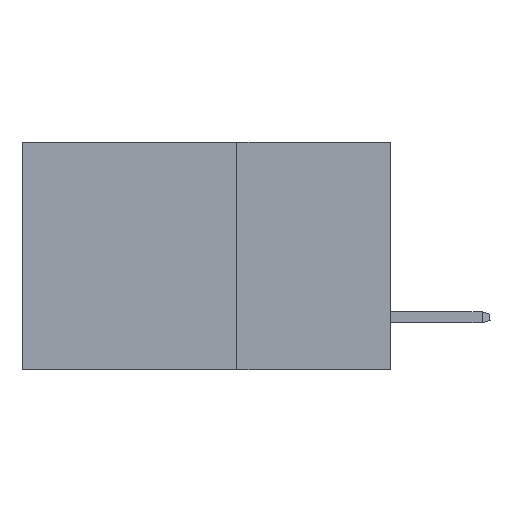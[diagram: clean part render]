
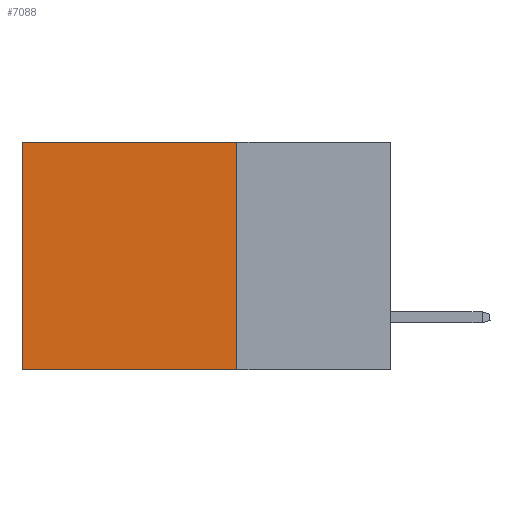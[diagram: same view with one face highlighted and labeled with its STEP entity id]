
A CAD part, left-side view. The second image highlights one B-rep face of the part: STEP entity #7088.
In plain terms, the highlighted planar face has unit normal (-1, 0, 0).
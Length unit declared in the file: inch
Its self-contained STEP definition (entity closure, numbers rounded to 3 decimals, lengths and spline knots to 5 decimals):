
#623 = CARTESIAN_POINT ( 'NONE',  ( 0.2875, 0.25, 0. ) ) ;
#876 = VECTOR ( 'NONE', #15731, 39.37008 ) ;
#918 = CARTESIAN_POINT ( 'NONE',  ( 0.2875, 0.25, 0. ) ) ;
#2680 = CARTESIAN_POINT ( 'NONE',  ( 0.2875, 0.6, 0. ) ) ;
#2746 = CARTESIAN_POINT ( 'NONE',  ( 0.2875, 0.6, -0.37 ) ) ;
#3376 = LINE ( 'NONE', #7480, #18117 ) ;
#4054 = VERTEX_POINT ( 'NONE', #22107 ) ;
#5449 = EDGE_CURVE ( 'NONE', #4054, #9744, #11555, .T. ) ;
#5782 = PLANE ( 'NONE',  #20547 ) ;
#7088 = ADVANCED_FACE ( 'NONE', ( #18167 ), #5782, .F. ) ;
#7453 = ORIENTED_EDGE ( 'NONE', *, *, #22435, .T. ) ;
#7480 = CARTESIAN_POINT ( 'NONE',  ( 0.2875, 0.25, 0. ) ) ;
#7561 = DIRECTION ( 'NONE',  ( 0., 0., -1. ) ) ;
#8186 = EDGE_CURVE ( 'NONE', #4054, #14778, #3376, .T. ) ;
#9525 = DIRECTION ( 'NONE',  ( 1., 0., 0. ) ) ;
#9744 = VERTEX_POINT ( 'NONE', #2680 ) ;
#11555 = LINE ( 'NONE', #918, #14645 ) ;
#12535 = ORIENTED_EDGE ( 'NONE', *, *, #5449, .T. ) ;
#13057 = DIRECTION ( 'NONE',  ( 0., 0., -1. ) ) ;
#13661 = VERTEX_POINT ( 'NONE', #2746 ) ;
#13965 = CARTESIAN_POINT ( 'NONE',  ( 0.2875, 0.25, -0.37 ) ) ;
#14645 = VECTOR ( 'NONE', #18710, 39.37008 ) ;
#14740 = CARTESIAN_POINT ( 'NONE',  ( 0.2875, 0.25, -0.37 ) ) ;
#14778 = VERTEX_POINT ( 'NONE', #14740 ) ;
#14921 = LINE ( 'NONE', #19357, #16280 ) ;
#15695 = DIRECTION ( 'NONE',  ( 0., 0., -1. ) ) ;
#15731 = DIRECTION ( 'NONE',  ( 0., 1., 0. ) ) ;
#16280 = VECTOR ( 'NONE', #15695, 39.37008 ) ;
#18117 = VECTOR ( 'NONE', #7561, 39.37008 ) ;
#18167 = FACE_OUTER_BOUND ( 'NONE', #22723, .T. ) ;
#18710 = DIRECTION ( 'NONE',  ( 0., 1., 0. ) ) ;
#18961 = EDGE_CURVE ( 'NONE', #14778, #13661, #21437, .T. ) ;
#19357 = CARTESIAN_POINT ( 'NONE',  ( 0.2875, 0.6, 0. ) ) ;
#20547 = AXIS2_PLACEMENT_3D ( 'NONE', #623, #9525, #13057 ) ;
#21437 = LINE ( 'NONE', #13965, #876 ) ;
#21941 = ORIENTED_EDGE ( 'NONE', *, *, #8186, .F. ) ;
#22107 = CARTESIAN_POINT ( 'NONE',  ( 0.2875, 0.25, 0. ) ) ;
#22343 = ORIENTED_EDGE ( 'NONE', *, *, #18961, .F. ) ;
#22435 = EDGE_CURVE ( 'NONE', #9744, #13661, #14921, .T. ) ;
#22723 = EDGE_LOOP ( 'NONE', ( #7453, #22343, #21941, #12535 ) ) ;
